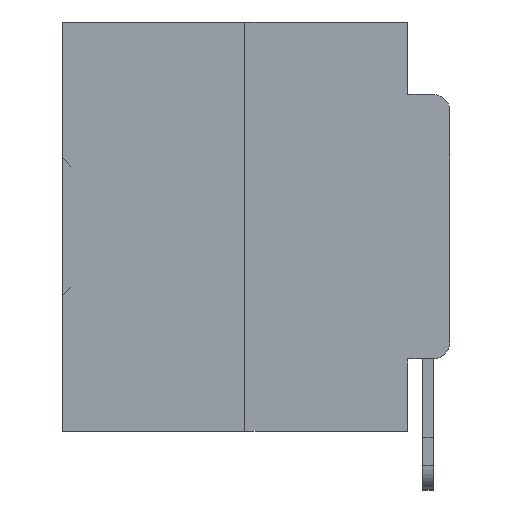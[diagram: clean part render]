
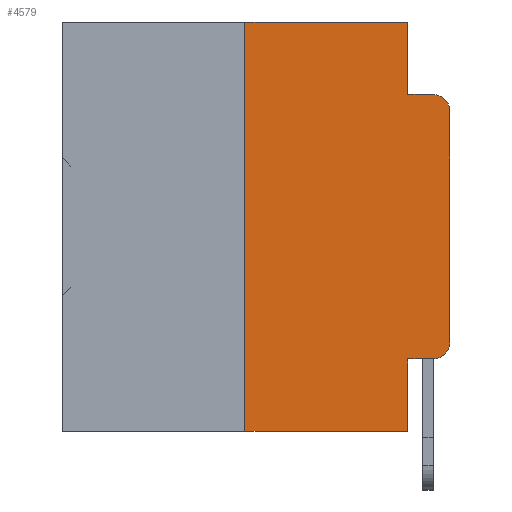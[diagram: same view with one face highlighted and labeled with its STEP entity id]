
A CAD part, left-side view. The second image highlights one B-rep face of the part: STEP entity #4579.
In plain terms, the highlighted planar face has unit normal (-1, 0, 0).
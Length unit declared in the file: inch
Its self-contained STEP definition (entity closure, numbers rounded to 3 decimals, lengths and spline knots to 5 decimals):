
#431 = CIRCLE ( 'NONE', #2289, 0.02 ) ;
#500 = DIRECTION ( 'NONE',  ( 0., 0., -1. ) ) ;
#1894 = VECTOR ( 'NONE', #17894, 39.37008 ) ;
#2289 = AXIS2_PLACEMENT_3D ( 'NONE', #22772, #4847, #25674 ) ;
#2347 = ORIENTED_EDGE ( 'NONE', *, *, #14909, .T. ) ;
#2889 = VERTEX_POINT ( 'NONE', #10756 ) ;
#4579 = ADVANCED_FACE ( 'NONE', ( #5405 ), #32933, .F. ) ;
#4616 = DIRECTION ( 'NONE',  ( 0., -1., 0. ) ) ;
#4847 = DIRECTION ( 'NONE',  ( -1., 0., 0. ) ) ;
#5175 = CARTESIAN_POINT ( 'NONE',  ( 0., 0.25, -0.5 ) ) ;
#5387 = VERTEX_POINT ( 'NONE', #28869 ) ;
#5405 = FACE_OUTER_BOUND ( 'NONE', #29808, .T. ) ;
#5623 = CARTESIAN_POINT ( 'NONE',  ( 0., 0.051, -0.4115 ) ) ;
#5884 = CARTESIAN_POINT ( 'NONE',  ( 0., 0.02, -0.4115 ) ) ;
#6165 = CARTESIAN_POINT ( 'NONE',  ( 0., 0., 0. ) ) ;
#6386 = CIRCLE ( 'NONE', #28286, 0.02 ) ;
#6837 = DIRECTION ( 'NONE',  ( 0., 0., -1. ) ) ;
#7119 = EDGE_CURVE ( 'NONE', #14562, #37467, #28290, .T. ) ;
#7162 = ORIENTED_EDGE ( 'NONE', *, *, #37365, .T. ) ;
#7265 = VECTOR ( 'NONE', #6837, 39.37008 ) ;
#8008 = VERTEX_POINT ( 'NONE', #32009 ) ;
#8720 = CARTESIAN_POINT ( 'NONE',  ( 0., 0.25, 0. ) ) ;
#9069 = CARTESIAN_POINT ( 'NONE',  ( 0., 0.473, 0. ) ) ;
#9430 = VERTEX_POINT ( 'NONE', #15174 ) ;
#9767 = VERTEX_POINT ( 'NONE', #5175 ) ;
#10063 = LINE ( 'NONE', #26779, #1894 ) ;
#10069 = VECTOR ( 'NONE', #26797, 39.37008 ) ;
#10497 = ORIENTED_EDGE ( 'NONE', *, *, #13331, .F. ) ;
#10756 = CARTESIAN_POINT ( 'NONE',  ( 0., 0.051, 0. ) ) ;
#11642 = EDGE_CURVE ( 'NONE', #13678, #2889, #31627, .T. ) ;
#12137 = VERTEX_POINT ( 'NONE', #5884 ) ;
#12179 = CARTESIAN_POINT ( 'NONE',  ( 0., 0.051, 0. ) ) ;
#12312 = VECTOR ( 'NONE', #4616, 39.37008 ) ;
#12518 = DIRECTION ( 'NONE',  ( -1., 0., 0. ) ) ;
#12644 = VECTOR ( 'NONE', #26906, 39.37008 ) ;
#13331 = EDGE_CURVE ( 'NONE', #9430, #5387, #19350, .T. ) ;
#13678 = VERTEX_POINT ( 'NONE', #8720 ) ;
#14562 = VERTEX_POINT ( 'NONE', #32115 ) ;
#14909 = EDGE_CURVE ( 'NONE', #37467, #5387, #431, .T. ) ;
#15127 = ORIENTED_EDGE ( 'NONE', *, *, #27147, .F. ) ;
#15174 = CARTESIAN_POINT ( 'NONE',  ( 0., 0.051, -0.0885 ) ) ;
#15222 = LINE ( 'NONE', #27395, #7265 ) ;
#15631 = CARTESIAN_POINT ( 'NONE',  ( 0., 0.473, 0. ) ) ;
#16078 = VECTOR ( 'NONE', #35254, 39.37008 ) ;
#16555 = CARTESIAN_POINT ( 'NONE',  ( 0., 0.473, -0.5 ) ) ;
#17894 = DIRECTION ( 'NONE',  ( 0., -1., 0. ) ) ;
#18378 = ORIENTED_EDGE ( 'NONE', *, *, #28118, .F. ) ;
#18603 = DIRECTION ( 'NONE',  ( 1., 0., 0. ) ) ;
#18871 = LINE ( 'NONE', #23907, #10069 ) ;
#19350 = LINE ( 'NONE', #27701, #33669 ) ;
#19933 = CARTESIAN_POINT ( 'NONE',  ( 0., 0., -0.1085 ) ) ;
#20221 = LINE ( 'NONE', #16555, #12312 ) ;
#20256 = ORIENTED_EDGE ( 'NONE', *, *, #11642, .F. ) ;
#22772 = CARTESIAN_POINT ( 'NONE',  ( 0., 0.02, -0.1085 ) ) ;
#23907 = CARTESIAN_POINT ( 'NONE',  ( 0., 0.25, 0. ) ) ;
#24009 = LINE ( 'NONE', #12179, #16078 ) ;
#24112 = VECTOR ( 'NONE', #32419, 39.37008 ) ;
#24577 = EDGE_CURVE ( 'NONE', #12137, #14562, #6386, .T. ) ;
#25674 = DIRECTION ( 'NONE',  ( 0., 0., -1. ) ) ;
#25676 = VERTEX_POINT ( 'NONE', #5623 ) ;
#25787 = EDGE_CURVE ( 'NONE', #25676, #12137, #10063, .T. ) ;
#26695 = ORIENTED_EDGE ( 'NONE', *, *, #24577, .T. ) ;
#26779 = CARTESIAN_POINT ( 'NONE',  ( 0., 0.051, -0.4115 ) ) ;
#26797 = DIRECTION ( 'NONE',  ( 0., 0., 1. ) ) ;
#26906 = DIRECTION ( 'NONE',  ( 0., 0., 1. ) ) ;
#27147 = EDGE_CURVE ( 'NONE', #25676, #8008, #15222, .T. ) ;
#27395 = CARTESIAN_POINT ( 'NONE',  ( 0., 0.051, 0. ) ) ;
#27701 = CARTESIAN_POINT ( 'NONE',  ( 0., 0.051, -0.0885 ) ) ;
#28064 = EDGE_CURVE ( 'NONE', #9767, #13678, #18871, .T. ) ;
#28118 = EDGE_CURVE ( 'NONE', #2889, #9430, #24009, .T. ) ;
#28286 = AXIS2_PLACEMENT_3D ( 'NONE', #30032, #12518, #32818 ) ;
#28290 = LINE ( 'NONE', #6165, #12644 ) ;
#28869 = CARTESIAN_POINT ( 'NONE',  ( 0., 0.02, -0.0885 ) ) ;
#29808 = EDGE_LOOP ( 'NONE', ( #37452, #2347, #10497, #18378, #20256, #35342, #7162, #15127, #32364, #26695 ) ) ;
#30032 = CARTESIAN_POINT ( 'NONE',  ( 0., 0.02, -0.3915 ) ) ;
#31627 = LINE ( 'NONE', #9069, #24112 ) ;
#32009 = CARTESIAN_POINT ( 'NONE',  ( 0., 0.051, -0.5 ) ) ;
#32115 = CARTESIAN_POINT ( 'NONE',  ( 0., 0., -0.3915 ) ) ;
#32364 = ORIENTED_EDGE ( 'NONE', *, *, #25787, .T. ) ;
#32419 = DIRECTION ( 'NONE',  ( 0., -1., 0. ) ) ;
#32818 = DIRECTION ( 'NONE',  ( 0., 0., -1. ) ) ;
#32933 = PLANE ( 'NONE',  #37108 ) ;
#33669 = VECTOR ( 'NONE', #36021, 39.37008 ) ;
#35254 = DIRECTION ( 'NONE',  ( 0., 0., -1. ) ) ;
#35342 = ORIENTED_EDGE ( 'NONE', *, *, #28064, .F. ) ;
#36021 = DIRECTION ( 'NONE',  ( 0., -1., 0. ) ) ;
#37108 = AXIS2_PLACEMENT_3D ( 'NONE', #15631, #18603, #500 ) ;
#37365 = EDGE_CURVE ( 'NONE', #9767, #8008, #20221, .T. ) ;
#37452 = ORIENTED_EDGE ( 'NONE', *, *, #7119, .T. ) ;
#37467 = VERTEX_POINT ( 'NONE', #19933 ) ;
